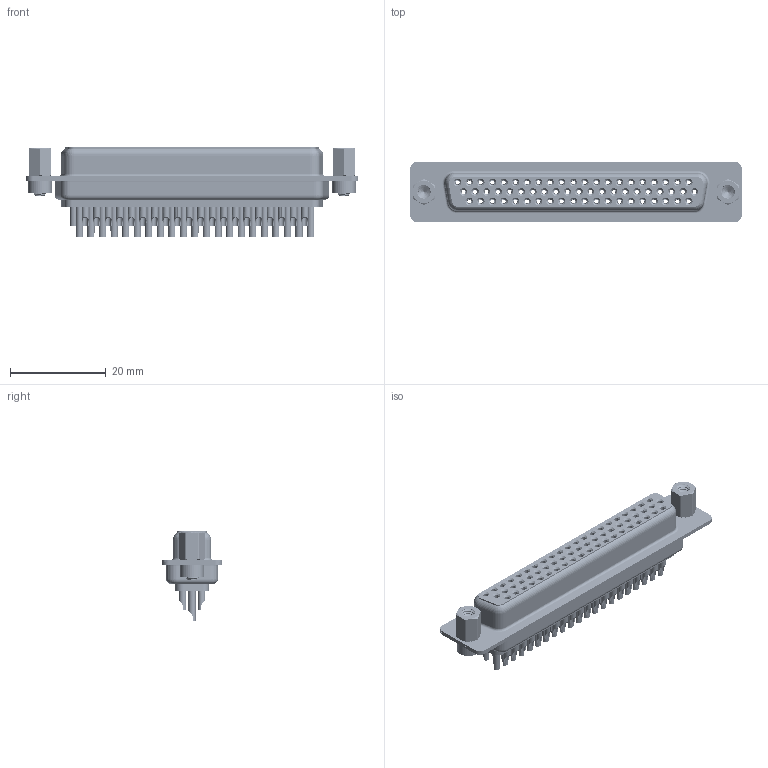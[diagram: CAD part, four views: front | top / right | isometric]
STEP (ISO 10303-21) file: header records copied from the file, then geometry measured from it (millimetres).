
FILE_DESCRIPTION (( 'STEP AP203' ), '1' );
FILE_NAME ('638-062-632-043.STEP', '2020-07-19T03:07:48', ( '' ), ( '' ), 'SwSTEP 2.0', 'SolidWorks 2020', '' );
FILE_SCHEMA (( 'CONFIG_CONTROL_DESIGN' ));
Length unit declared in the file: millimetre
Products named in the file (9): 638 4-40 Hex Standoff; 638 Housing_62 Contacts; 638 Contact Row 2_32; 638-062-632-043; 638 Shell Front_62 Contacts; 638 Shell Rear_62 Contacts; 638 Contact Row 3_32; 638 Contact Row 1_32; 638 4-40 Threaded Rivet
Assembly tree (69 placements, depth 2):
  638-062-632-043
    638 Housing_62 Contacts
    638 Shell Front_62 Contacts
    638 Shell Rear_62 Contacts
    638 Contact Row 1_32  x21
    638 Contact Row 2_32  x21
    638 Contact Row 3_32  x20
    638 4-40 Threaded Rivet  x2
    638 4-40 Hex Standoff  x2
Bounding box: 69.32 x 12.6 x 18.6 mm (x, y, z)
Volume: 4922.7 mm3; surface area: 19036.7 mm2
Topology: 69 solids, 69 shells, 5923 faces, 15045 edges, 9457 vertices
Faces by surface type: cylinder 1759, plane 1391, bspline 1258, torus 1173, cone 342
Entity records: 47935 total; most frequent: CARTESIAN_POINT 13912, DIRECTION 7022, ORIENTED_EDGE 6212, EDGE_CURVE 3106, AXIS2_PLACEMENT_3D 2969, VERTEX_POINT 1976, EDGE_LOOP 1678, CIRCLE 1623
